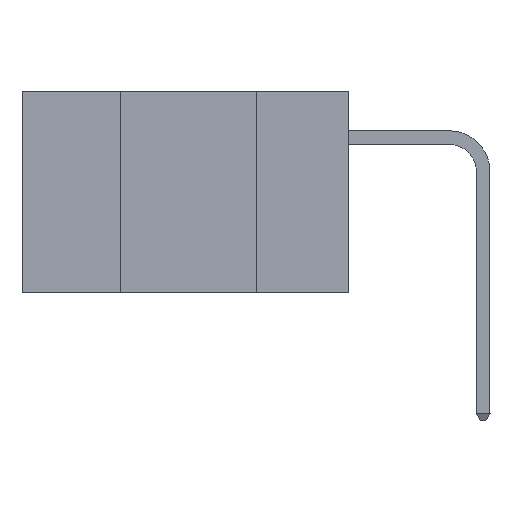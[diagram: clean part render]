
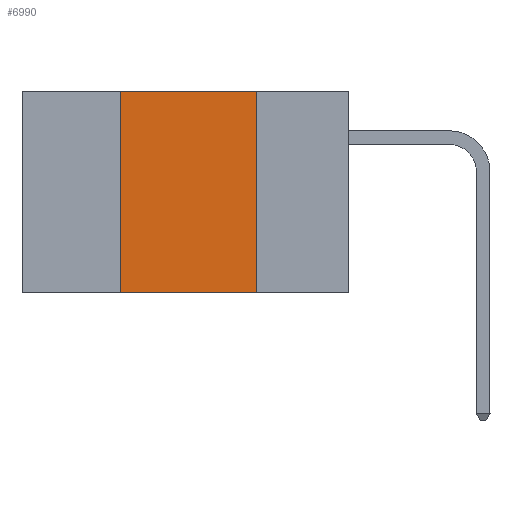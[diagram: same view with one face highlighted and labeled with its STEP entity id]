
A CAD part, left-side view. The second image highlights one B-rep face of the part: STEP entity #6990.
In plain terms, the highlighted planar face has unit normal (-1, 0, 0).
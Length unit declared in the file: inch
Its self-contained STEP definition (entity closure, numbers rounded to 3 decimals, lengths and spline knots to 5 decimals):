
#402 = ORIENTED_EDGE ( 'NONE', *, *, #8255, .T. ) ;
#550 = VERTEX_POINT ( 'NONE', #36378 ) ;
#618 = VECTOR ( 'NONE', #35816, 39.37008 ) ;
#1020 = ORIENTED_EDGE ( 'NONE', *, *, #34507, .F. ) ;
#2471 = VERTEX_POINT ( 'NONE', #18659 ) ;
#2917 = CARTESIAN_POINT ( 'NONE',  ( 0., 0.6, 0. ) ) ;
#3553 = DIRECTION ( 'NONE',  ( 0., -1., 0. ) ) ;
#3892 = ORIENTED_EDGE ( 'NONE', *, *, #15228, .F. ) ;
#6425 = DIRECTION ( 'NONE',  ( 1., 0., 0. ) ) ;
#6479 = VECTOR ( 'NONE', #34254, 39.37008 ) ;
#6828 = LINE ( 'NONE', #39537, #28556 ) ;
#6990 = ADVANCED_FACE ( 'NONE', ( #22442 ), #19132, .F. ) ;
#8255 = EDGE_CURVE ( 'NONE', #11949, #550, #39996, .T. ) ;
#10624 = CARTESIAN_POINT ( 'NONE',  ( 0., 0.17, 0. ) ) ;
#11949 = VERTEX_POINT ( 'NONE', #39533 ) ;
#12422 = AXIS2_PLACEMENT_3D ( 'NONE', #2917, #6425, #12980 ) ;
#12980 = DIRECTION ( 'NONE',  ( 0., 0., -1. ) ) ;
#13629 = CARTESIAN_POINT ( 'NONE',  ( 0., 0.17, 0. ) ) ;
#15228 = EDGE_CURVE ( 'NONE', #32272, #550, #30312, .T. ) ;
#18090 = VECTOR ( 'NONE', #33417, 39.37008 ) ;
#18659 = CARTESIAN_POINT ( 'NONE',  ( 0., 0.42, 0. ) ) ;
#19132 = PLANE ( 'NONE',  #12422 ) ;
#20692 = CARTESIAN_POINT ( 'NONE',  ( 0., 0.42, 0. ) ) ;
#22442 = FACE_OUTER_BOUND ( 'NONE', #29694, .T. ) ;
#22660 = CARTESIAN_POINT ( 'NONE',  ( 0., 0.6, -0.37 ) ) ;
#28556 = VECTOR ( 'NONE', #3553, 39.37008 ) ;
#29694 = EDGE_LOOP ( 'NONE', ( #3892, #1020, #38952, #402 ) ) ;
#30312 = LINE ( 'NONE', #13629, #6479 ) ;
#32272 = VERTEX_POINT ( 'NONE', #10624 ) ;
#33417 = DIRECTION ( 'NONE',  ( 0., 0., 1. ) ) ;
#34254 = DIRECTION ( 'NONE',  ( 0., 0., -1. ) ) ;
#34507 = EDGE_CURVE ( 'NONE', #2471, #32272, #6828, .T. ) ;
#35353 = EDGE_CURVE ( 'NONE', #11949, #2471, #36928, .T. ) ;
#35816 = DIRECTION ( 'NONE',  ( 0., -1., 0. ) ) ;
#36378 = CARTESIAN_POINT ( 'NONE',  ( 0., 0.17, -0.37 ) ) ;
#36928 = LINE ( 'NONE', #20692, #18090 ) ;
#38952 = ORIENTED_EDGE ( 'NONE', *, *, #35353, .F. ) ;
#39533 = CARTESIAN_POINT ( 'NONE',  ( 0., 0.42, -0.37 ) ) ;
#39537 = CARTESIAN_POINT ( 'NONE',  ( 0., 0.6, 0. ) ) ;
#39996 = LINE ( 'NONE', #22660, #618 ) ;
